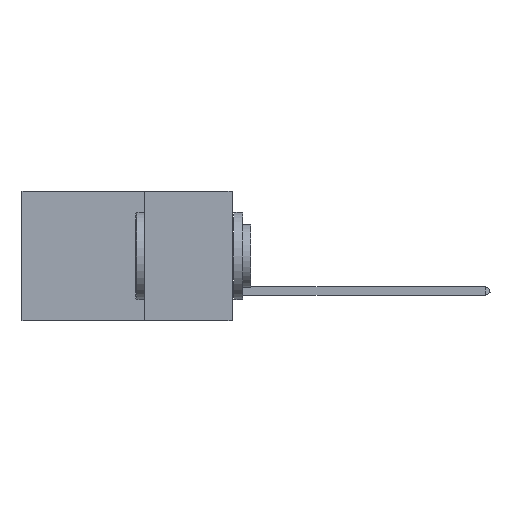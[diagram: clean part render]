
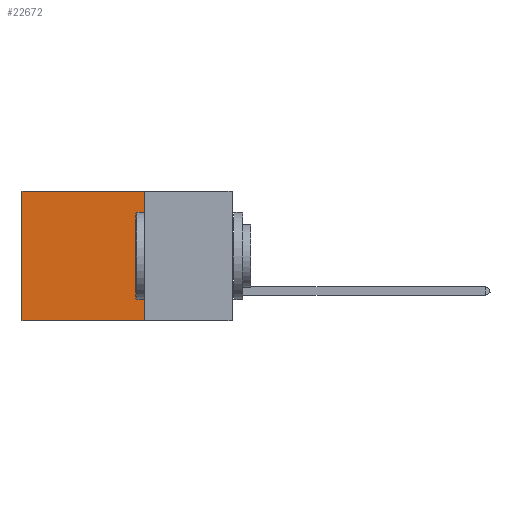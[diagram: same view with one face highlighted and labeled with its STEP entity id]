
A CAD part, left-side view. The second image highlights one B-rep face of the part: STEP entity #22672.
In plain terms, the highlighted planar face has unit normal (-1, 0, 0).
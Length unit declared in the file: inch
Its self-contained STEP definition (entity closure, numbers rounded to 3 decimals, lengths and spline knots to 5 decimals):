
#2174 = DIRECTION ( 'NONE',  ( 0., 0., -1. ) ) ;
#2258 = DIRECTION ( 'NONE',  ( 1., 0., 0. ) ) ;
#3067 = CARTESIAN_POINT ( 'NONE',  ( 0.2875, 0.25, 0. ) ) ;
#3367 = VERTEX_POINT ( 'NONE', #16946 ) ;
#6089 = CARTESIAN_POINT ( 'NONE',  ( 0.2875, 0.25, -0.37 ) ) ;
#6901 = VECTOR ( 'NONE', #19650, 39.37008 ) ;
#6910 = CARTESIAN_POINT ( 'NONE',  ( 0.2875, 0.6, 0. ) ) ;
#7395 = ORIENTED_EDGE ( 'NONE', *, *, #14435, .F. ) ;
#7500 = DIRECTION ( 'NONE',  ( 0., 0., -1. ) ) ;
#8337 = CARTESIAN_POINT ( 'NONE',  ( 0.2875, 0.25, 0. ) ) ;
#8644 = LINE ( 'NONE', #8337, #28746 ) ;
#8708 = FACE_OUTER_BOUND ( 'NONE', #18878, .T. ) ;
#9009 = EDGE_CURVE ( 'NONE', #3367, #28075, #18213, .T. ) ;
#9620 = ORIENTED_EDGE ( 'NONE', *, *, #10009, .T. ) ;
#9676 = AXIS2_PLACEMENT_3D ( 'NONE', #24728, #2258, #2174 ) ;
#10009 = EDGE_CURVE ( 'NONE', #23328, #23709, #8644, .T. ) ;
#11085 = PLANE ( 'NONE',  #9676 ) ;
#12677 = DIRECTION ( 'NONE',  ( 0., 0., -1. ) ) ;
#13283 = DIRECTION ( 'NONE',  ( 0., 1., 0. ) ) ;
#14243 = ORIENTED_EDGE ( 'NONE', *, *, #9009, .F. ) ;
#14435 = EDGE_CURVE ( 'NONE', #23328, #3367, #27600, .T. ) ;
#15209 = ORIENTED_EDGE ( 'NONE', *, *, #27468, .T. ) ;
#15766 = CARTESIAN_POINT ( 'NONE',  ( 0.2875, 0.25, 0. ) ) ;
#16539 = CARTESIAN_POINT ( 'NONE',  ( 0.2875, 0.6, 0. ) ) ;
#16946 = CARTESIAN_POINT ( 'NONE',  ( 0.2875, 0.25, -0.37 ) ) ;
#18213 = LINE ( 'NONE', #6089, #6901 ) ;
#18878 = EDGE_LOOP ( 'NONE', ( #15209, #14243, #7395, #9620 ) ) ;
#19650 = DIRECTION ( 'NONE',  ( 0., 1., 0. ) ) ;
#20468 = VECTOR ( 'NONE', #7500, 39.37008 ) ;
#20892 = CARTESIAN_POINT ( 'NONE',  ( 0.2875, 0.6, -0.37 ) ) ;
#22672 = ADVANCED_FACE ( 'NONE', ( #8708 ), #11085, .F. ) ;
#23328 = VERTEX_POINT ( 'NONE', #15766 ) ;
#23709 = VERTEX_POINT ( 'NONE', #16539 ) ;
#24728 = CARTESIAN_POINT ( 'NONE',  ( 0.2875, 0.25, 0. ) ) ;
#24734 = LINE ( 'NONE', #6910, #20468 ) ;
#25886 = VECTOR ( 'NONE', #12677, 39.37008 ) ;
#27468 = EDGE_CURVE ( 'NONE', #23709, #28075, #24734, .T. ) ;
#27600 = LINE ( 'NONE', #3067, #25886 ) ;
#28075 = VERTEX_POINT ( 'NONE', #20892 ) ;
#28746 = VECTOR ( 'NONE', #13283, 39.37008 ) ;
